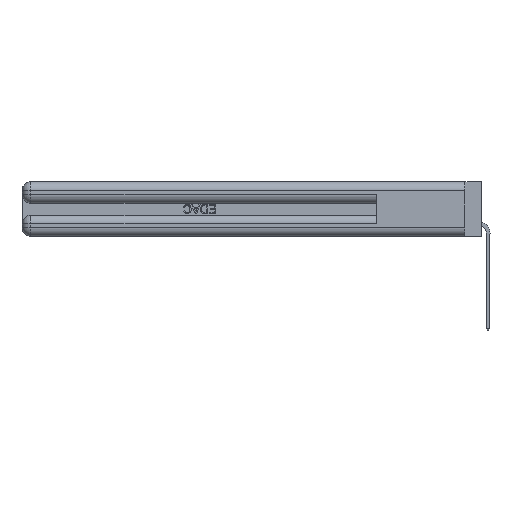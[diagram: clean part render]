
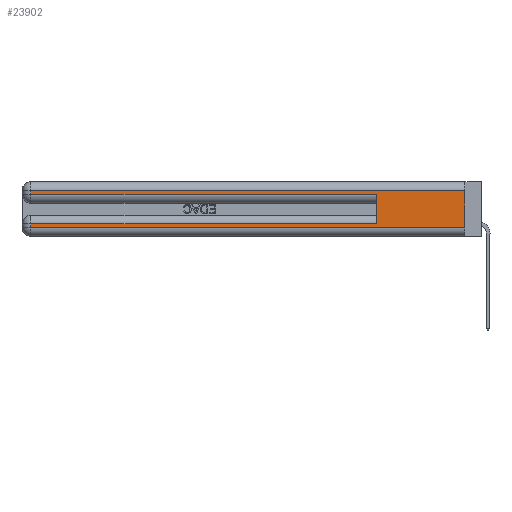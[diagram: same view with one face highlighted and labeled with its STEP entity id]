
A CAD part, left-side view. The second image highlights one B-rep face of the part: STEP entity #23902.
In plain terms, the highlighted planar face has unit normal (-1, 0, 0).
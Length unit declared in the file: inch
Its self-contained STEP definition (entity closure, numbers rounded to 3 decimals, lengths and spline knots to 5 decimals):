
#692 = LINE ( 'NONE', #14262, #16281 ) ;
#847 = VERTEX_POINT ( 'NONE', #27849 ) ;
#1055 = DIRECTION ( 'NONE',  ( 0., 1., 0. ) ) ;
#1682 = LINE ( 'NONE', #15496, #15960 ) ;
#2644 = CARTESIAN_POINT ( 'NONE',  ( 0., 2.94, 0.085 ) ) ;
#3120 = VERTEX_POINT ( 'NONE', #27775 ) ;
#3663 = VERTEX_POINT ( 'NONE', #35546 ) ;
#3850 = LINE ( 'NONE', #34240, #32782 ) ;
#4109 = VECTOR ( 'NONE', #20787, 39.37008 ) ;
#4845 = CARTESIAN_POINT ( 'NONE',  ( 0., 0., 0.285 ) ) ;
#5102 = ORIENTED_EDGE ( 'NONE', *, *, #17784, .F. ) ;
#5654 = CARTESIAN_POINT ( 'NONE',  ( 0., 0., 0.085 ) ) ;
#5659 = EDGE_CURVE ( 'NONE', #25048, #847, #31319, .T. ) ;
#5784 = EDGE_LOOP ( 'NONE', ( #23025, #21587, #20759, #12276, #5102, #29124, #12901, #15634 ) ) ;
#5786 = VERTEX_POINT ( 'NONE', #2644 ) ;
#6239 = LINE ( 'NONE', #21146, #4109 ) ;
#6727 = EDGE_CURVE ( 'NONE', #29884, #25048, #6239, .T. ) ;
#7987 = DIRECTION ( 'NONE',  ( 0., -1., 0. ) ) ;
#8046 = CARTESIAN_POINT ( 'NONE',  ( 0., 2.94, 0.06 ) ) ;
#8931 = EDGE_CURVE ( 'NONE', #3663, #34846, #19934, .T. ) ;
#10491 = EDGE_CURVE ( 'NONE', #5786, #34233, #1682, .T. ) ;
#10692 = PLANE ( 'NONE',  #35273 ) ;
#11519 = EDGE_CURVE ( 'NONE', #34233, #34846, #692, .T. ) ;
#11812 = LINE ( 'NONE', #5654, #35588 ) ;
#12276 = ORIENTED_EDGE ( 'NONE', *, *, #5659, .T. ) ;
#12552 = LINE ( 'NONE', #23498, #15986 ) ;
#12901 = ORIENTED_EDGE ( 'NONE', *, *, #10491, .T. ) ;
#14262 = CARTESIAN_POINT ( 'NONE',  ( 0., 0., 0.06 ) ) ;
#15496 = CARTESIAN_POINT ( 'NONE',  ( 0., 2.94, 0.37 ) ) ;
#15634 = ORIENTED_EDGE ( 'NONE', *, *, #11519, .T. ) ;
#15646 = VECTOR ( 'NONE', #21073, 39.37008 ) ;
#15960 = VECTOR ( 'NONE', #32123, 39.37008 ) ;
#15986 = VECTOR ( 'NONE', #1055, 39.37008 ) ;
#16281 = VECTOR ( 'NONE', #34053, 39.37008 ) ;
#17774 = EDGE_CURVE ( 'NONE', #3663, #29884, #12552, .T. ) ;
#17784 = EDGE_CURVE ( 'NONE', #3120, #847, #3850, .T. ) ;
#18560 = CARTESIAN_POINT ( 'NONE',  ( 0., 0., 0.37 ) ) ;
#19934 = LINE ( 'NONE', #27026, #15646 ) ;
#20745 = FACE_OUTER_BOUND ( 'NONE', #5784, .T. ) ;
#20759 = ORIENTED_EDGE ( 'NONE', *, *, #6727, .T. ) ;
#20787 = DIRECTION ( 'NONE',  ( 0., 0., -1. ) ) ;
#21073 = DIRECTION ( 'NONE',  ( 0., 0., -1. ) ) ;
#21146 = CARTESIAN_POINT ( 'NONE',  ( 0., 2.94, 0.37 ) ) ;
#21587 = ORIENTED_EDGE ( 'NONE', *, *, #17774, .T. ) ;
#21813 = EDGE_CURVE ( 'NONE', #3120, #5786, #11812, .T. ) ;
#22444 = DIRECTION ( 'NONE',  ( 0., 1., 0. ) ) ;
#23025 = ORIENTED_EDGE ( 'NONE', *, *, #8931, .F. ) ;
#23239 = CARTESIAN_POINT ( 'NONE',  ( 0., 2.94, 0.31 ) ) ;
#23498 = CARTESIAN_POINT ( 'NONE',  ( 0., 0., 0.31 ) ) ;
#23902 = ADVANCED_FACE ( 'NONE', ( #20745 ), #10692, .F. ) ;
#24030 = VECTOR ( 'NONE', #7987, 39.37008 ) ;
#25048 = VERTEX_POINT ( 'NONE', #32205 ) ;
#27026 = CARTESIAN_POINT ( 'NONE',  ( 0., 0., 0.37 ) ) ;
#27274 = CARTESIAN_POINT ( 'NONE',  ( 0., 0., 0.06 ) ) ;
#27775 = CARTESIAN_POINT ( 'NONE',  ( 0., 0.6, 0.085 ) ) ;
#27849 = CARTESIAN_POINT ( 'NONE',  ( 0., 0.6, 0.285 ) ) ;
#29124 = ORIENTED_EDGE ( 'NONE', *, *, #21813, .T. ) ;
#29479 = DIRECTION ( 'NONE',  ( 0., 0., -1. ) ) ;
#29884 = VERTEX_POINT ( 'NONE', #23239 ) ;
#31319 = LINE ( 'NONE', #4845, #24030 ) ;
#32123 = DIRECTION ( 'NONE',  ( 0., 0., -1. ) ) ;
#32205 = CARTESIAN_POINT ( 'NONE',  ( 0., 2.94, 0.285 ) ) ;
#32757 = DIRECTION ( 'NONE',  ( 1., 0., 0. ) ) ;
#32782 = VECTOR ( 'NONE', #34632, 39.37008 ) ;
#34053 = DIRECTION ( 'NONE',  ( 0., -1., 0. ) ) ;
#34233 = VERTEX_POINT ( 'NONE', #8046 ) ;
#34240 = CARTESIAN_POINT ( 'NONE',  ( 0., 0.6, 0.145 ) ) ;
#34632 = DIRECTION ( 'NONE',  ( 0., 0., 1. ) ) ;
#34846 = VERTEX_POINT ( 'NONE', #27274 ) ;
#35273 = AXIS2_PLACEMENT_3D ( 'NONE', #18560, #32757, #29479 ) ;
#35546 = CARTESIAN_POINT ( 'NONE',  ( 0., 0., 0.31 ) ) ;
#35588 = VECTOR ( 'NONE', #22444, 39.37008 ) ;
